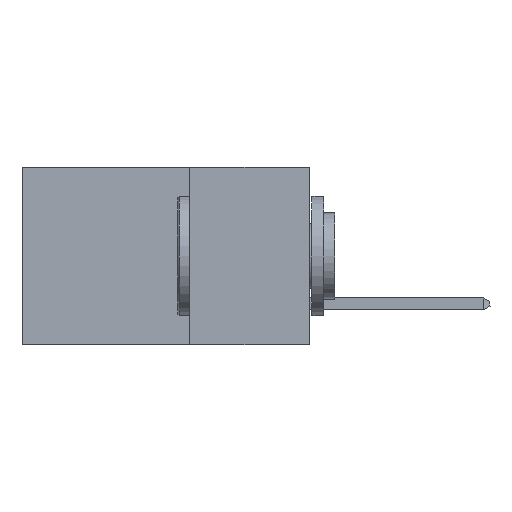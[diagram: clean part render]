
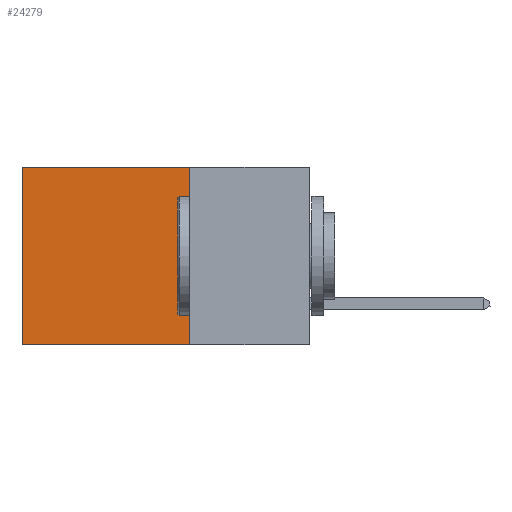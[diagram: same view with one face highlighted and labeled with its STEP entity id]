
A CAD part, left-side view. The second image highlights one B-rep face of the part: STEP entity #24279.
In plain terms, the highlighted planar face has unit normal (-1, 0, 0).
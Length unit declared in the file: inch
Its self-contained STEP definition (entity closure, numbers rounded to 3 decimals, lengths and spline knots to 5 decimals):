
#767 = LINE ( 'NONE', #13237, #7753 ) ;
#1460 = EDGE_CURVE ( 'NONE', #31360, #31449, #767, .T. ) ;
#4873 = ORIENTED_EDGE ( 'NONE', *, *, #19284, .F. ) ;
#5766 = DIRECTION ( 'NONE',  ( 0., 1., 0. ) ) ;
#5838 = AXIS2_PLACEMENT_3D ( 'NONE', #13461, #16456, #37169 ) ;
#7054 = LINE ( 'NONE', #13876, #20967 ) ;
#7753 = VECTOR ( 'NONE', #16229, 39.37008 ) ;
#10389 = ORIENTED_EDGE ( 'NONE', *, *, #1460, .T. ) ;
#11238 = LINE ( 'NONE', #11648, #33015 ) ;
#11648 = CARTESIAN_POINT ( 'NONE',  ( 0.2875, 0.25, -0.37 ) ) ;
#13237 = CARTESIAN_POINT ( 'NONE',  ( 0.2875, 0.25, 0. ) ) ;
#13461 = CARTESIAN_POINT ( 'NONE',  ( 0.2875, 0.25, 0. ) ) ;
#13876 = CARTESIAN_POINT ( 'NONE',  ( 0.2875, 0.25, 0. ) ) ;
#16229 = DIRECTION ( 'NONE',  ( 0., 1., 0. ) ) ;
#16456 = DIRECTION ( 'NONE',  ( 1., 0., 0. ) ) ;
#16866 = DIRECTION ( 'NONE',  ( 0., 0., -1. ) ) ;
#17364 = ORIENTED_EDGE ( 'NONE', *, *, #18533, .F. ) ;
#18533 = EDGE_CURVE ( 'NONE', #31360, #32394, #7054, .T. ) ;
#19284 = EDGE_CURVE ( 'NONE', #32394, #31375, #11238, .T. ) ;
#20967 = VECTOR ( 'NONE', #16866, 39.37008 ) ;
#21064 = CARTESIAN_POINT ( 'NONE',  ( 0.2875, 0.25, -0.37 ) ) ;
#21675 = CARTESIAN_POINT ( 'NONE',  ( 0.2875, 0.6, -0.37 ) ) ;
#22995 = EDGE_CURVE ( 'NONE', #31449, #31375, #36873, .T. ) ;
#23131 = ORIENTED_EDGE ( 'NONE', *, *, #22995, .T. ) ;
#24279 = ADVANCED_FACE ( 'NONE', ( #26110 ), #31194, .F. ) ;
#25247 = DIRECTION ( 'NONE',  ( 0., 0., -1. ) ) ;
#25292 = CARTESIAN_POINT ( 'NONE',  ( 0.2875, 0.6, 0. ) ) ;
#26110 = FACE_OUTER_BOUND ( 'NONE', #35410, .T. ) ;
#27480 = CARTESIAN_POINT ( 'NONE',  ( 0.2875, 0.25, 0. ) ) ;
#28964 = VECTOR ( 'NONE', #25247, 39.37008 ) ;
#31194 = PLANE ( 'NONE',  #5838 ) ;
#31360 = VERTEX_POINT ( 'NONE', #27480 ) ;
#31375 = VERTEX_POINT ( 'NONE', #21675 ) ;
#31449 = VERTEX_POINT ( 'NONE', #25292 ) ;
#32394 = VERTEX_POINT ( 'NONE', #21064 ) ;
#33015 = VECTOR ( 'NONE', #5766, 39.37008 ) ;
#35410 = EDGE_LOOP ( 'NONE', ( #23131, #4873, #17364, #10389 ) ) ;
#36873 = LINE ( 'NONE', #37038, #28964 ) ;
#37038 = CARTESIAN_POINT ( 'NONE',  ( 0.2875, 0.6, 0. ) ) ;
#37169 = DIRECTION ( 'NONE',  ( 0., 0., -1. ) ) ;
